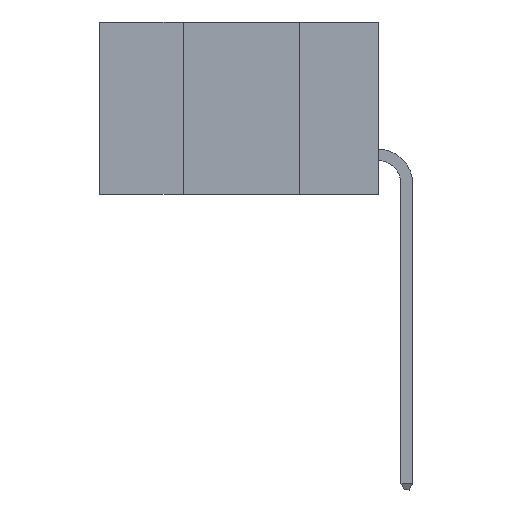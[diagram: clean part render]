
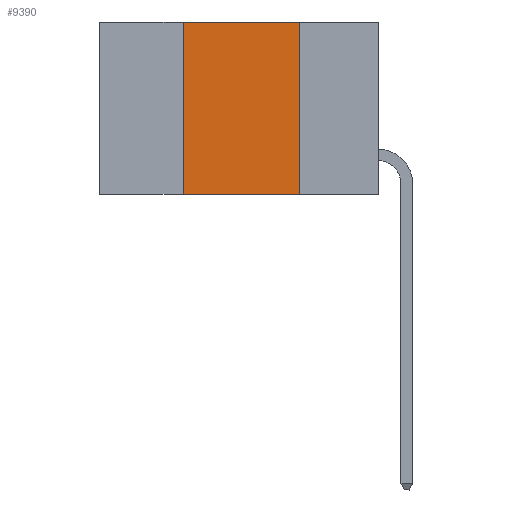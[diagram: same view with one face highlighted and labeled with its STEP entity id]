
A CAD part, left-side view. The second image highlights one B-rep face of the part: STEP entity #9390.
In plain terms, the highlighted planar face has unit normal (-1, 0, 0).
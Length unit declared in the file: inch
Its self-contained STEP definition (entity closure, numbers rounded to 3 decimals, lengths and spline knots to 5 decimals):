
#430 = FACE_OUTER_BOUND ( 'NONE', #4273, .T. ) ;
#623 = EDGE_CURVE ( 'NONE', #2259, #6871, #12758, .T. ) ;
#792 = CARTESIAN_POINT ( 'NONE',  ( 0., 0.17, 0. ) ) ;
#845 = VERTEX_POINT ( 'NONE', #1718 ) ;
#1618 = LINE ( 'NONE', #4362, #12792 ) ;
#1718 = CARTESIAN_POINT ( 'NONE',  ( 0., 0.42, -0.37 ) ) ;
#2259 = VERTEX_POINT ( 'NONE', #792 ) ;
#3870 = VECTOR ( 'NONE', #11107, 39.37008 ) ;
#4097 = DIRECTION ( 'NONE',  ( 0., 0., 1. ) ) ;
#4169 = DIRECTION ( 'NONE',  ( 1., 0., 0. ) ) ;
#4238 = VECTOR ( 'NONE', #4097, 39.37008 ) ;
#4273 = EDGE_LOOP ( 'NONE', ( #9671, #10644, #10495, #8466 ) ) ;
#4362 = CARTESIAN_POINT ( 'NONE',  ( 0., 0.6, -0.37 ) ) ;
#5235 = CARTESIAN_POINT ( 'NONE',  ( 0., 0.42, 0. ) ) ;
#6871 = VERTEX_POINT ( 'NONE', #7720 ) ;
#7720 = CARTESIAN_POINT ( 'NONE',  ( 0., 0.17, -0.37 ) ) ;
#8466 = ORIENTED_EDGE ( 'NONE', *, *, #9506, .T. ) ;
#9124 = EDGE_CURVE ( 'NONE', #9235, #2259, #9504, .T. ) ;
#9204 = CARTESIAN_POINT ( 'NONE',  ( 0., 0.42, 0. ) ) ;
#9233 = AXIS2_PLACEMENT_3D ( 'NONE', #13411, #4169, #11492 ) ;
#9235 = VERTEX_POINT ( 'NONE', #9204 ) ;
#9390 = ADVANCED_FACE ( 'NONE', ( #430 ), #9453, .F. ) ;
#9453 = PLANE ( 'NONE',  #9233 ) ;
#9463 = VECTOR ( 'NONE', #12783, 39.37008 ) ;
#9504 = LINE ( 'NONE', #12107, #3870 ) ;
#9506 = EDGE_CURVE ( 'NONE', #845, #6871, #1618, .T. ) ;
#9671 = ORIENTED_EDGE ( 'NONE', *, *, #623, .F. ) ;
#10495 = ORIENTED_EDGE ( 'NONE', *, *, #11551, .F. ) ;
#10644 = ORIENTED_EDGE ( 'NONE', *, *, #9124, .F. ) ;
#10662 = DIRECTION ( 'NONE',  ( 0., -1., 0. ) ) ;
#11107 = DIRECTION ( 'NONE',  ( 0., -1., 0. ) ) ;
#11492 = DIRECTION ( 'NONE',  ( 0., 0., -1. ) ) ;
#11551 = EDGE_CURVE ( 'NONE', #845, #9235, #12535, .T. ) ;
#11800 = CARTESIAN_POINT ( 'NONE',  ( 0., 0.17, 0. ) ) ;
#12107 = CARTESIAN_POINT ( 'NONE',  ( 0., 0.6, 0. ) ) ;
#12535 = LINE ( 'NONE', #5235, #4238 ) ;
#12758 = LINE ( 'NONE', #11800, #9463 ) ;
#12783 = DIRECTION ( 'NONE',  ( 0., 0., -1. ) ) ;
#12792 = VECTOR ( 'NONE', #10662, 39.37008 ) ;
#13411 = CARTESIAN_POINT ( 'NONE',  ( 0., 0.6, 0. ) ) ;
